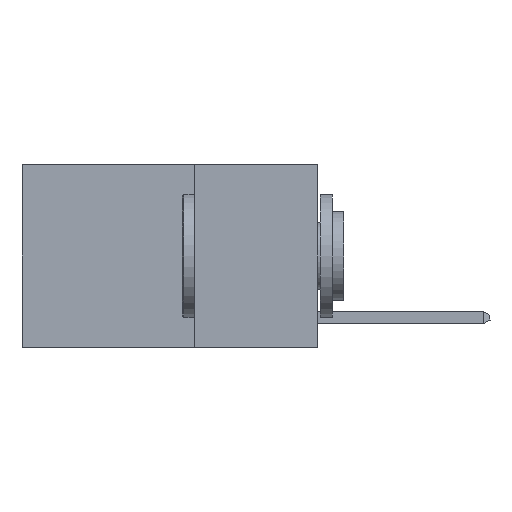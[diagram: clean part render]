
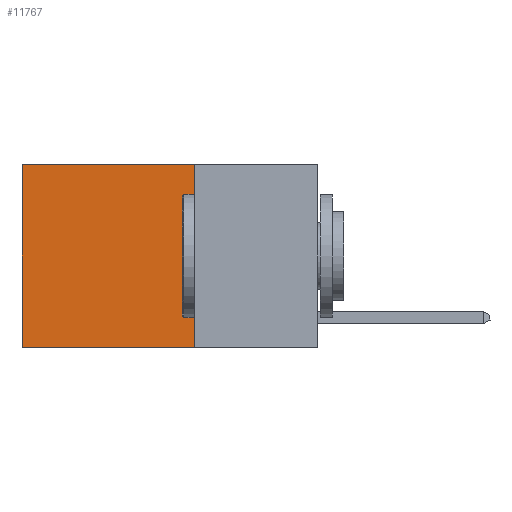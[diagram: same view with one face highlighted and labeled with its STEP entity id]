
A CAD part, left-side view. The second image highlights one B-rep face of the part: STEP entity #11767.
In plain terms, the highlighted planar face has unit normal (-1, 0, 0).
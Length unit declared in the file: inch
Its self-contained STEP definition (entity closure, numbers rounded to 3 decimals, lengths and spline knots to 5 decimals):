
#188 = EDGE_CURVE ( 'NONE', #15486, #1836, #9576, .T. ) ;
#412 = EDGE_CURVE ( 'NONE', #2111, #9434, #6897, .T. ) ;
#850 = CARTESIAN_POINT ( 'NONE',  ( 0.2625, 0.6, 0. ) ) ;
#993 = CARTESIAN_POINT ( 'NONE',  ( 0.2625, 0.6, 0. ) ) ;
#1703 = DIRECTION ( 'NONE',  ( 1., 0., 0. ) ) ;
#1836 = VERTEX_POINT ( 'NONE', #993 ) ;
#2111 = VERTEX_POINT ( 'NONE', #8821 ) ;
#2437 = EDGE_CURVE ( 'NONE', #1836, #9434, #16762, .T. ) ;
#3196 = DIRECTION ( 'NONE',  ( 0., 0., -1. ) ) ;
#3770 = FACE_OUTER_BOUND ( 'NONE', #16282, .T. ) ;
#4150 = ORIENTED_EDGE ( 'NONE', *, *, #10341, .F. ) ;
#5343 = ORIENTED_EDGE ( 'NONE', *, *, #2437, .T. ) ;
#5775 = VECTOR ( 'NONE', #8992, 39.37008 ) ;
#5952 = VECTOR ( 'NONE', #15154, 39.37008 ) ;
#6035 = PLANE ( 'NONE',  #12062 ) ;
#6897 = LINE ( 'NONE', #14512, #13531 ) ;
#7433 = VECTOR ( 'NONE', #3196, 39.37008 ) ;
#8821 = CARTESIAN_POINT ( 'NONE',  ( 0.2625, 0.25, -0.37 ) ) ;
#8992 = DIRECTION ( 'NONE',  ( 0., 1., 0. ) ) ;
#9434 = VERTEX_POINT ( 'NONE', #15248 ) ;
#9576 = LINE ( 'NONE', #10392, #5775 ) ;
#10341 = EDGE_CURVE ( 'NONE', #15486, #2111, #11240, .T. ) ;
#10392 = CARTESIAN_POINT ( 'NONE',  ( 0.2625, 0.25, 0. ) ) ;
#11240 = LINE ( 'NONE', #13137, #7433 ) ;
#11767 = ADVANCED_FACE ( 'NONE', ( #3770 ), #6035, .F. ) ;
#11783 = DIRECTION ( 'NONE',  ( 0., 0., -1. ) ) ;
#12062 = AXIS2_PLACEMENT_3D ( 'NONE', #14519, #1703, #11783 ) ;
#12638 = ORIENTED_EDGE ( 'NONE', *, *, #188, .T. ) ;
#13137 = CARTESIAN_POINT ( 'NONE',  ( 0.2625, 0.25, 0. ) ) ;
#13294 = DIRECTION ( 'NONE',  ( 0., 1., 0. ) ) ;
#13531 = VECTOR ( 'NONE', #13294, 39.37008 ) ;
#14512 = CARTESIAN_POINT ( 'NONE',  ( 0.2625, 0.25, -0.37 ) ) ;
#14519 = CARTESIAN_POINT ( 'NONE',  ( 0.2625, 0.25, 0. ) ) ;
#15154 = DIRECTION ( 'NONE',  ( 0., 0., -1. ) ) ;
#15248 = CARTESIAN_POINT ( 'NONE',  ( 0.2625, 0.6, -0.37 ) ) ;
#15414 = CARTESIAN_POINT ( 'NONE',  ( 0.2625, 0.25, 0. ) ) ;
#15486 = VERTEX_POINT ( 'NONE', #15414 ) ;
#16282 = EDGE_LOOP ( 'NONE', ( #5343, #17462, #4150, #12638 ) ) ;
#16762 = LINE ( 'NONE', #850, #5952 ) ;
#17462 = ORIENTED_EDGE ( 'NONE', *, *, #412, .F. ) ;
